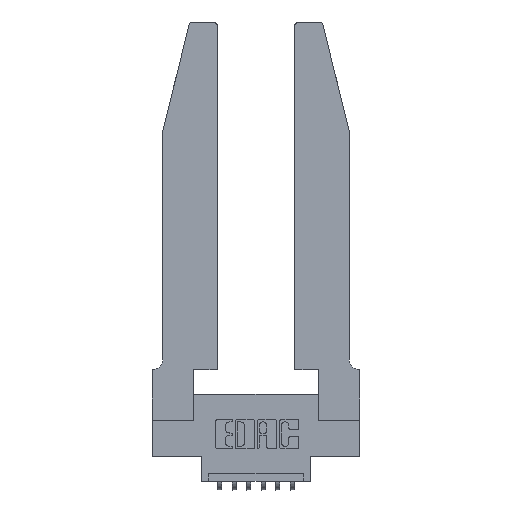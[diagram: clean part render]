
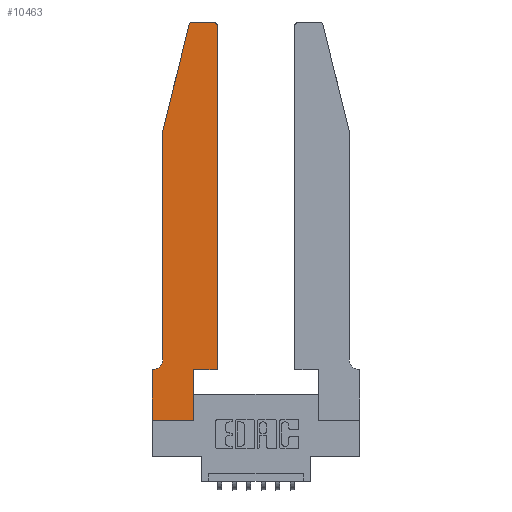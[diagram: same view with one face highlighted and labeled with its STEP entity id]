
A CAD part, top view. The second image highlights one B-rep face of the part: STEP entity #10463.
In plain terms, the highlighted planar face has unit normal (0, 0, 1).
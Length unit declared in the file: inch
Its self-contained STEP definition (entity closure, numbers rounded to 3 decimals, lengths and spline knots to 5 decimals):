
#42 = EDGE_CURVE ( 'NONE', #12561, #13753, #10570, .T. ) ;
#126 = EDGE_CURVE ( 'NONE', #2694, #11523, #12136, .T. ) ;
#155 = AXIS2_PLACEMENT_3D ( 'NONE', #9687, #5027, #12813 ) ;
#241 = VERTEX_POINT ( 'NONE', #743 ) ;
#646 = CARTESIAN_POINT ( 'NONE',  ( 0., 0., 0.37 ) ) ;
#743 = CARTESIAN_POINT ( 'NONE',  ( 0.2865, 0.35, 0.37 ) ) ;
#1216 = LINE ( 'NONE', #7322, #2068 ) ;
#1463 = CIRCLE ( 'NONE', #155, 0.03 ) ;
#1595 = AXIS2_PLACEMENT_3D ( 'NONE', #6673, #8814, #4582 ) ;
#1739 = DIRECTION ( 'NONE',  ( 1., 0., 0. ) ) ;
#1791 = DIRECTION ( 'NONE',  ( -1., 0., 0. ) ) ;
#2045 = VECTOR ( 'NONE', #10999, 39.37008 ) ;
#2068 = VECTOR ( 'NONE', #4123, 39.37008 ) ;
#2438 = EDGE_CURVE ( 'NONE', #11523, #7072, #9747, .T. ) ;
#2694 = VERTEX_POINT ( 'NONE', #9859 ) ;
#2840 = FACE_OUTER_BOUND ( 'NONE', #7341, .T. ) ;
#3383 = VECTOR ( 'NONE', #13471, 39.37008 ) ;
#3561 = ORIENTED_EDGE ( 'NONE', *, *, #2438, .T. ) ;
#3601 = CARTESIAN_POINT ( 'NONE',  ( 0.0755, 2., 0.37 ) ) ;
#3674 = EDGE_CURVE ( 'NONE', #12250, #4725, #9526, .T. ) ;
#3683 = CARTESIAN_POINT ( 'NONE',  ( 0.25487, 2.72718, 0.37 ) ) ;
#3740 = ORIENTED_EDGE ( 'NONE', *, *, #8265, .T. ) ;
#3779 = CARTESIAN_POINT ( 'NONE',  ( 0.0755, 0.35, 0.37 ) ) ;
#3813 = EDGE_CURVE ( 'NONE', #241, #7032, #3954, .T. ) ;
#3904 = CARTESIAN_POINT ( 'NONE',  ( 0., 0.35, 0.37 ) ) ;
#3954 = LINE ( 'NONE', #10946, #12501 ) ;
#4091 = AXIS2_PLACEMENT_3D ( 'NONE', #5116, #11725, #8368 ) ;
#4123 = DIRECTION ( 'NONE',  ( -0.239, -0.971, 0. ) ) ;
#4206 = CARTESIAN_POINT ( 'NONE',  ( 0.4205, 2.75, 0.37 ) ) ;
#4442 = CIRCLE ( 'NONE', #4091, 0.03 ) ;
#4582 = DIRECTION ( 'NONE',  ( -1., 0., 0. ) ) ;
#4609 = CARTESIAN_POINT ( 'NONE',  ( 0.4505, 0.35, 0.37 ) ) ;
#4725 = VERTEX_POINT ( 'NONE', #6381 ) ;
#4839 = VECTOR ( 'NONE', #1791, 39.37008 ) ;
#4936 = PLANE ( 'NONE',  #6795 ) ;
#5027 = DIRECTION ( 'NONE',  ( 0., 0., 1. ) ) ;
#5052 = ORIENTED_EDGE ( 'NONE', *, *, #10388, .T. ) ;
#5116 = CARTESIAN_POINT ( 'NONE',  ( 0.4205, 2.72, 0.37 ) ) ;
#5262 = EDGE_CURVE ( 'NONE', #13930, #12561, #1216, .T. ) ;
#5857 = CARTESIAN_POINT ( 'NONE',  ( 0.2865, 0., 0.37 ) ) ;
#6130 = ORIENTED_EDGE ( 'NONE', *, *, #10301, .T. ) ;
#6131 = DIRECTION ( 'NONE',  ( 0., -1., 0. ) ) ;
#6381 = CARTESIAN_POINT ( 'NONE',  ( 0.284, 2.75, 0.37 ) ) ;
#6521 = CARTESIAN_POINT ( 'NONE',  ( 0.2865, 0.35, 0.37 ) ) ;
#6594 = EDGE_CURVE ( 'NONE', #13753, #8951, #9119, .T. ) ;
#6673 = CARTESIAN_POINT ( 'NONE',  ( 0.0055, 0.42, 0.37 ) ) ;
#6786 = ORIENTED_EDGE ( 'NONE', *, *, #9524, .T. ) ;
#6795 = AXIS2_PLACEMENT_3D ( 'NONE', #3904, #7205, #12571 ) ;
#6947 = VECTOR ( 'NONE', #1739, 39.37008 ) ;
#7032 = VERTEX_POINT ( 'NONE', #11212 ) ;
#7072 = VERTEX_POINT ( 'NONE', #5857 ) ;
#7114 = ORIENTED_EDGE ( 'NONE', *, *, #8655, .T. ) ;
#7205 = DIRECTION ( 'NONE',  ( 0., 0., 1. ) ) ;
#7322 = CARTESIAN_POINT ( 'NONE',  ( 0.0755, 2., 0.37 ) ) ;
#7341 = EDGE_LOOP ( 'NONE', ( #13098, #5052, #8768, #9757, #12118, #6130, #12717, #3561, #3740, #10048, #6786, #7114 ) ) ;
#8106 = DIRECTION ( 'NONE',  ( 0., -1., 0. ) ) ;
#8265 = EDGE_CURVE ( 'NONE', #7072, #241, #10536, .T. ) ;
#8368 = DIRECTION ( 'NONE',  ( 1., 0., 0. ) ) ;
#8635 = VECTOR ( 'NONE', #6131, 39.37008 ) ;
#8655 = EDGE_CURVE ( 'NONE', #10476, #12250, #4442, .T. ) ;
#8768 = ORIENTED_EDGE ( 'NONE', *, *, #5262, .T. ) ;
#8814 = DIRECTION ( 'NONE',  ( 0., 0., -1. ) ) ;
#8951 = VERTEX_POINT ( 'NONE', #12021 ) ;
#9119 = CIRCLE ( 'NONE', #1595, 0.07 ) ;
#9524 = EDGE_CURVE ( 'NONE', #7032, #10476, #9810, .T. ) ;
#9526 = LINE ( 'NONE', #12553, #4839 ) ;
#9553 = CARTESIAN_POINT ( 'NONE',  ( 0., 0., 0.37 ) ) ;
#9687 = CARTESIAN_POINT ( 'NONE',  ( 0.284, 2.72, 0.37 ) ) ;
#9747 = LINE ( 'NONE', #13895, #6947 ) ;
#9757 = ORIENTED_EDGE ( 'NONE', *, *, #42, .T. ) ;
#9810 = LINE ( 'NONE', #4609, #3383 ) ;
#9859 = CARTESIAN_POINT ( 'NONE',  ( 0., 0.35, 0.37 ) ) ;
#10048 = ORIENTED_EDGE ( 'NONE', *, *, #3813, .T. ) ;
#10116 = CARTESIAN_POINT ( 'NONE',  ( 0.0755, 2., 0.37 ) ) ;
#10301 = EDGE_CURVE ( 'NONE', #8951, #2694, #14318, .T. ) ;
#10388 = EDGE_CURVE ( 'NONE', #4725, #13930, #1463, .T. ) ;
#10463 = ADVANCED_FACE ( 'NONE', ( #2840 ), #4936, .T. ) ;
#10476 = VERTEX_POINT ( 'NONE', #14165 ) ;
#10536 = LINE ( 'NONE', #6521, #2045 ) ;
#10570 = LINE ( 'NONE', #3601, #13195 ) ;
#10946 = CARTESIAN_POINT ( 'NONE',  ( 0.4505, 0.35, 0.37 ) ) ;
#10996 = DIRECTION ( 'NONE',  ( 1., 0., 0. ) ) ;
#10999 = DIRECTION ( 'NONE',  ( 0., 1., 0. ) ) ;
#11187 = VECTOR ( 'NONE', #13668, 39.37008 ) ;
#11212 = CARTESIAN_POINT ( 'NONE',  ( 0.4505, 0.35, 0.37 ) ) ;
#11317 = CARTESIAN_POINT ( 'NONE',  ( 0.0755, 0.42, 0.37 ) ) ;
#11523 = VERTEX_POINT ( 'NONE', #9553 ) ;
#11725 = DIRECTION ( 'NONE',  ( 0., 0., 1. ) ) ;
#12021 = CARTESIAN_POINT ( 'NONE',  ( 0.0055, 0.35, 0.37 ) ) ;
#12118 = ORIENTED_EDGE ( 'NONE', *, *, #6594, .T. ) ;
#12136 = LINE ( 'NONE', #646, #8635 ) ;
#12250 = VERTEX_POINT ( 'NONE', #4206 ) ;
#12501 = VECTOR ( 'NONE', #10996, 39.37008 ) ;
#12553 = CARTESIAN_POINT ( 'NONE',  ( 0.2605, 2.75, 0.37 ) ) ;
#12561 = VERTEX_POINT ( 'NONE', #10116 ) ;
#12571 = DIRECTION ( 'NONE',  ( 1., 0., 0. ) ) ;
#12717 = ORIENTED_EDGE ( 'NONE', *, *, #126, .T. ) ;
#12813 = DIRECTION ( 'NONE',  ( 1., 0., 0. ) ) ;
#13098 = ORIENTED_EDGE ( 'NONE', *, *, #3674, .T. ) ;
#13195 = VECTOR ( 'NONE', #8106, 39.37008 ) ;
#13471 = DIRECTION ( 'NONE',  ( 0., 1., 0. ) ) ;
#13668 = DIRECTION ( 'NONE',  ( -1., 0., 0. ) ) ;
#13753 = VERTEX_POINT ( 'NONE', #11317 ) ;
#13895 = CARTESIAN_POINT ( 'NONE',  ( 0., 0., 0.37 ) ) ;
#13930 = VERTEX_POINT ( 'NONE', #3683 ) ;
#14165 = CARTESIAN_POINT ( 'NONE',  ( 0.4505, 2.72, 0.37 ) ) ;
#14318 = LINE ( 'NONE', #3779, #11187 ) ;
